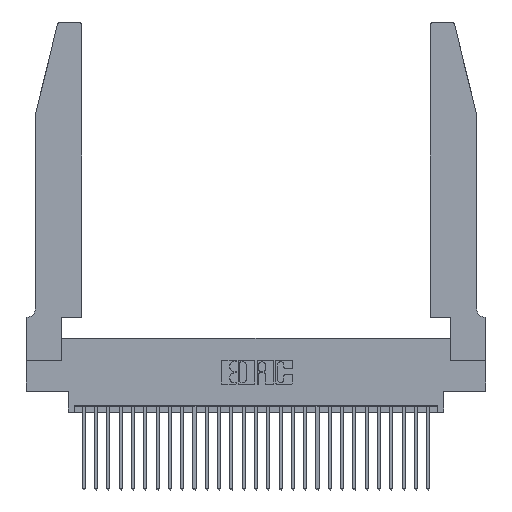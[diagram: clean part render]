
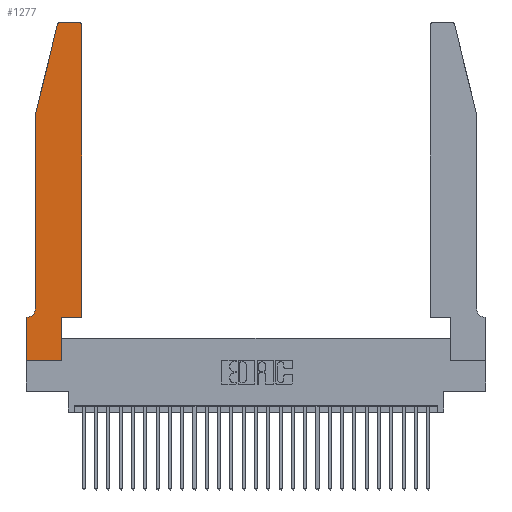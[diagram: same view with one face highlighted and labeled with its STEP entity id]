
A CAD part, top view. The second image highlights one B-rep face of the part: STEP entity #1277.
In plain terms, the highlighted planar face has unit normal (0, 0, 1).
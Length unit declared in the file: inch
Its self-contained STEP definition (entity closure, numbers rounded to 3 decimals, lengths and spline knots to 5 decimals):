
#221 = VECTOR ( 'NONE', #5533, 39.37008 ) ;
#260 = DIRECTION ( 'NONE',  ( -1., 0., 0. ) ) ;
#1150 = CARTESIAN_POINT ( 'NONE',  ( 0.25487, 2.72718, 0.37 ) ) ;
#1261 = ORIENTED_EDGE ( 'NONE', *, *, #2530, .T. ) ;
#1277 = ADVANCED_FACE ( 'NONE', ( #26104 ), #22198, .T. ) ;
#1716 = VERTEX_POINT ( 'NONE', #2809 ) ;
#1804 = VERTEX_POINT ( 'NONE', #17822 ) ;
#1851 = VERTEX_POINT ( 'NONE', #27248 ) ;
#2036 = EDGE_CURVE ( 'NONE', #21363, #1851, #29344, .T. ) ;
#2241 = DIRECTION ( 'NONE',  ( 1., 0., 0. ) ) ;
#2423 = EDGE_CURVE ( 'NONE', #1716, #6741, #20179, .T. ) ;
#2530 = EDGE_CURVE ( 'NONE', #13793, #1804, #5260, .T. ) ;
#2619 = CARTESIAN_POINT ( 'NONE',  ( 0., 0., 0.37 ) ) ;
#2698 = LINE ( 'NONE', #2619, #26116 ) ;
#2809 = CARTESIAN_POINT ( 'NONE',  ( 0.0755, 2., 0.37 ) ) ;
#3181 = VECTOR ( 'NONE', #5597, 39.37008 ) ;
#3240 = VECTOR ( 'NONE', #20032, 39.37008 ) ;
#3272 = CARTESIAN_POINT ( 'NONE',  ( 0., 0., 0.37 ) ) ;
#3859 = ORIENTED_EDGE ( 'NONE', *, *, #28308, .T. ) ;
#4181 = EDGE_CURVE ( 'NONE', #1804, #26717, #17606, .T. ) ;
#4425 = ORIENTED_EDGE ( 'NONE', *, *, #21753, .T. ) ;
#5260 = CIRCLE ( 'NONE', #19763, 0.03 ) ;
#5533 = DIRECTION ( 'NONE',  ( -0.239, -0.971, 0. ) ) ;
#5597 = DIRECTION ( 'NONE',  ( 1., 0., 0. ) ) ;
#6741 = VERTEX_POINT ( 'NONE', #15022 ) ;
#7033 = EDGE_CURVE ( 'NONE', #18918, #27839, #16791, .T. ) ;
#7244 = VERTEX_POINT ( 'NONE', #14315 ) ;
#9370 = LINE ( 'NONE', #10953, #3240 ) ;
#9970 = CARTESIAN_POINT ( 'NONE',  ( 0.284, 2.75, 0.37 ) ) ;
#10251 = ORIENTED_EDGE ( 'NONE', *, *, #13662, .T. ) ;
#10728 = CARTESIAN_POINT ( 'NONE',  ( 0.4505, 0.35, 0.37 ) ) ;
#10953 = CARTESIAN_POINT ( 'NONE',  ( 0.4505, 0.35, 0.37 ) ) ;
#11003 = DIRECTION ( 'NONE',  ( 0., 0., 1. ) ) ;
#11043 = DIRECTION ( 'NONE',  ( 1., 0., 0. ) ) ;
#11074 = CARTESIAN_POINT ( 'NONE',  ( 0.4205, 2.72, 0.37 ) ) ;
#11091 = CIRCLE ( 'NONE', #28184, 0.07 ) ;
#11140 = ORIENTED_EDGE ( 'NONE', *, *, #7033, .T. ) ;
#11292 = VECTOR ( 'NONE', #11581, 39.37008 ) ;
#11463 = VECTOR ( 'NONE', #24828, 39.37008 ) ;
#11581 = DIRECTION ( 'NONE',  ( -1., 0., 0. ) ) ;
#11583 = VECTOR ( 'NONE', #20873, 39.37008 ) ;
#12400 = AXIS2_PLACEMENT_3D ( 'NONE', #24508, #14032, #14192 ) ;
#12657 = EDGE_CURVE ( 'NONE', #1851, #28652, #9370, .T. ) ;
#12792 = CARTESIAN_POINT ( 'NONE',  ( 0.4505, 2.72, 0.37 ) ) ;
#13510 = VECTOR ( 'NONE', #16395, 39.37008 ) ;
#13662 = EDGE_CURVE ( 'NONE', #7244, #21363, #21342, .T. ) ;
#13793 = VERTEX_POINT ( 'NONE', #12792 ) ;
#14031 = DIRECTION ( 'NONE',  ( 0., 0., -1. ) ) ;
#14032 = DIRECTION ( 'NONE',  ( 0., 0., 1. ) ) ;
#14089 = CARTESIAN_POINT ( 'NONE',  ( 0.4505, 0.35, 0.37 ) ) ;
#14192 = DIRECTION ( 'NONE',  ( 1., 0., 0. ) ) ;
#14315 = CARTESIAN_POINT ( 'NONE',  ( 0., 0., 0.37 ) ) ;
#14344 = ORIENTED_EDGE ( 'NONE', *, *, #15661, .T. ) ;
#14536 = ORIENTED_EDGE ( 'NONE', *, *, #14750, .T. ) ;
#14750 = EDGE_CURVE ( 'NONE', #22002, #1716, #28299, .T. ) ;
#14819 = AXIS2_PLACEMENT_3D ( 'NONE', #29409, #15963, #2241 ) ;
#15022 = CARTESIAN_POINT ( 'NONE',  ( 0.0755, 0.42, 0.37 ) ) ;
#15661 = EDGE_CURVE ( 'NONE', #28652, #13793, #17591, .T. ) ;
#15963 = DIRECTION ( 'NONE',  ( 0., 0., 1. ) ) ;
#16395 = DIRECTION ( 'NONE',  ( 0., -1., 0. ) ) ;
#16791 = LINE ( 'NONE', #29347, #11463 ) ;
#17591 = LINE ( 'NONE', #14089, #11583 ) ;
#17606 = LINE ( 'NONE', #22829, #11292 ) ;
#17674 = CARTESIAN_POINT ( 'NONE',  ( 0.2865, 0.35, 0.37 ) ) ;
#17822 = CARTESIAN_POINT ( 'NONE',  ( 0.4205, 2.75, 0.37 ) ) ;
#18168 = ORIENTED_EDGE ( 'NONE', *, *, #20563, .T. ) ;
#18187 = DIRECTION ( 'NONE',  ( 0., 1., 0. ) ) ;
#18918 = VERTEX_POINT ( 'NONE', #20379 ) ;
#19145 = CARTESIAN_POINT ( 'NONE',  ( 0.0755, 2., 0.37 ) ) ;
#19744 = ORIENTED_EDGE ( 'NONE', *, *, #2423, .T. ) ;
#19763 = AXIS2_PLACEMENT_3D ( 'NONE', #11074, #11003, #11043 ) ;
#20032 = DIRECTION ( 'NONE',  ( 1., 0., 0. ) ) ;
#20179 = LINE ( 'NONE', #27211, #13510 ) ;
#20379 = CARTESIAN_POINT ( 'NONE',  ( 0.0055, 0.35, 0.37 ) ) ;
#20508 = ORIENTED_EDGE ( 'NONE', *, *, #2036, .T. ) ;
#20563 = EDGE_CURVE ( 'NONE', #26717, #22002, #21931, .T. ) ;
#20873 = DIRECTION ( 'NONE',  ( 0., 1., 0. ) ) ;
#21342 = LINE ( 'NONE', #3272, #3181 ) ;
#21363 = VERTEX_POINT ( 'NONE', #25727 ) ;
#21753 = EDGE_CURVE ( 'NONE', #6741, #18918, #11091, .T. ) ;
#21931 = CIRCLE ( 'NONE', #14819, 0.03 ) ;
#22002 = VERTEX_POINT ( 'NONE', #1150 ) ;
#22198 = PLANE ( 'NONE',  #12400 ) ;
#22679 = VECTOR ( 'NONE', #18187, 39.37008 ) ;
#22829 = CARTESIAN_POINT ( 'NONE',  ( 0.2605, 2.75, 0.37 ) ) ;
#23108 = DIRECTION ( 'NONE',  ( 0., -1., 0. ) ) ;
#23564 = ORIENTED_EDGE ( 'NONE', *, *, #4181, .T. ) ;
#23808 = CARTESIAN_POINT ( 'NONE',  ( 0., 0.35, 0.37 ) ) ;
#24508 = CARTESIAN_POINT ( 'NONE',  ( 0., 0.35, 0.37 ) ) ;
#24828 = DIRECTION ( 'NONE',  ( -1., 0., 0. ) ) ;
#24976 = ORIENTED_EDGE ( 'NONE', *, *, #12657, .T. ) ;
#25727 = CARTESIAN_POINT ( 'NONE',  ( 0.2865, 0., 0.37 ) ) ;
#26104 = FACE_OUTER_BOUND ( 'NONE', #28678, .T. ) ;
#26116 = VECTOR ( 'NONE', #23108, 39.37008 ) ;
#26717 = VERTEX_POINT ( 'NONE', #9970 ) ;
#27211 = CARTESIAN_POINT ( 'NONE',  ( 0.0755, 2., 0.37 ) ) ;
#27248 = CARTESIAN_POINT ( 'NONE',  ( 0.2865, 0.35, 0.37 ) ) ;
#27490 = CARTESIAN_POINT ( 'NONE',  ( 0.0055, 0.42, 0.37 ) ) ;
#27839 = VERTEX_POINT ( 'NONE', #23808 ) ;
#28184 = AXIS2_PLACEMENT_3D ( 'NONE', #27490, #14031, #260 ) ;
#28299 = LINE ( 'NONE', #19145, #221 ) ;
#28308 = EDGE_CURVE ( 'NONE', #27839, #7244, #2698, .T. ) ;
#28652 = VERTEX_POINT ( 'NONE', #10728 ) ;
#28678 = EDGE_LOOP ( 'NONE', ( #23564, #18168, #14536, #19744, #4425, #11140, #3859, #10251, #20508, #24976, #14344, #1261 ) ) ;
#29344 = LINE ( 'NONE', #17674, #22679 ) ;
#29347 = CARTESIAN_POINT ( 'NONE',  ( 0.0755, 0.35, 0.37 ) ) ;
#29409 = CARTESIAN_POINT ( 'NONE',  ( 0.284, 2.72, 0.37 ) ) ;
